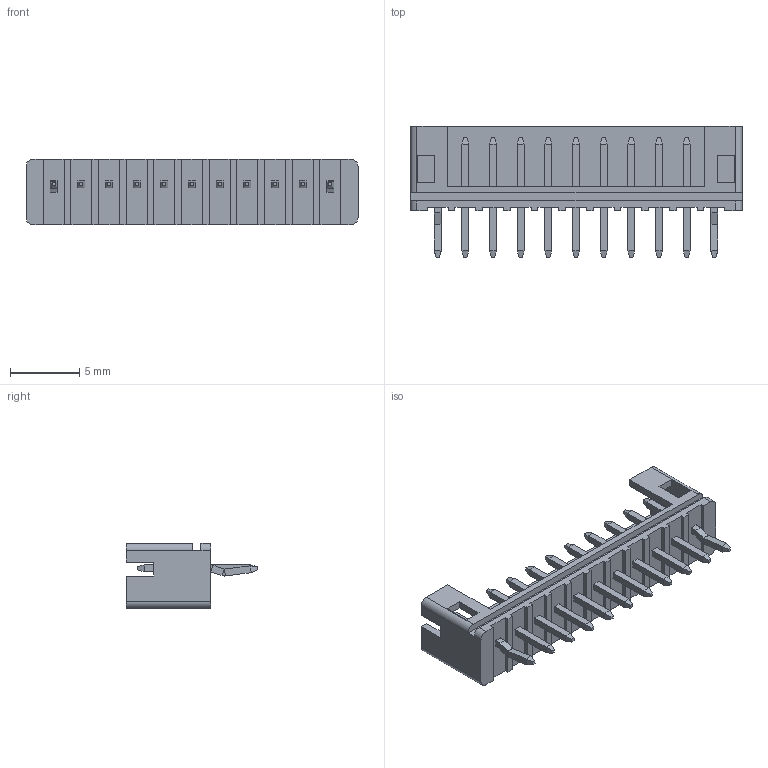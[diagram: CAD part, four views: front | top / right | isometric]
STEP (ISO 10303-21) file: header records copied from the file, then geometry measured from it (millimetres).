
FILE_DESCRIPTION (( 'STEP AP203' ), '1' );
FILE_NAME ('140-511-415-001.STEP', '2020-03-31T19:24:37', ( '' ), ( '' ), 'SwSTEP 2.0', 'SolidWorks 2016', '' );
FILE_SCHEMA (( 'CONFIG_CONTROL_DESIGN' ));
Length unit declared in the file: millimetre
Products named in the file (4): V Contact_Str; 140-511-415-001; V Housing_511; V Contact_Kink
Assembly tree (12 placements, depth 2):
  140-511-415-001
    V Housing_511
    V Contact_Kink  x2
    V Contact_Str  x9
Bounding box: 24 x 9.51 x 4.7 mm (x, y, z)
Volume: 251.3 mm3; surface area: 918.4 mm2
Topology: 12 solids, 12 shells, 312 faces, 758 edges, 468 vertices
Faces by surface type: plane 294, cylinder 16, bspline 2
Entity records: 6095 total; most frequent: CARTESIAN_POINT 996, ORIENTED_EDGE 942, DIRECTION 865, EDGE_CURVE 471, VECTOR 447, LINE 447, VERTEX_POINT 304, AXIS2_PLACEMENT_3D 209
